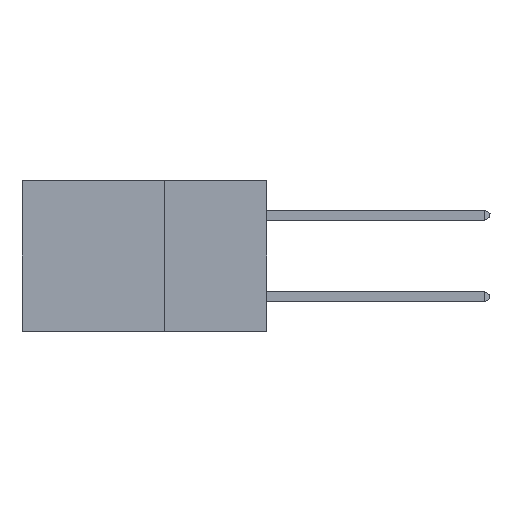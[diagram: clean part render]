
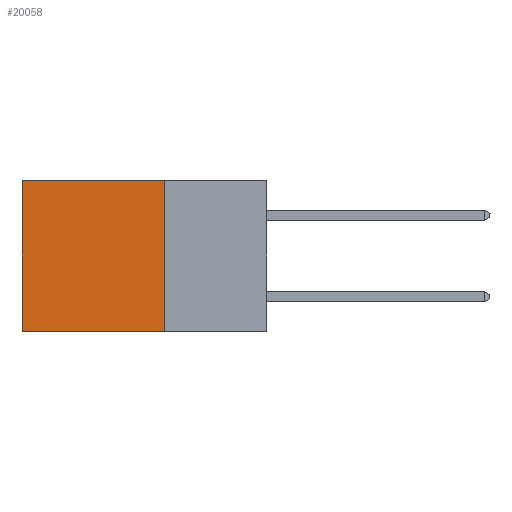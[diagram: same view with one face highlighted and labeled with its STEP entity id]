
A CAD part, left-side view. The second image highlights one B-rep face of the part: STEP entity #20058.
In plain terms, the highlighted planar face has unit normal (-1, 0, 0).
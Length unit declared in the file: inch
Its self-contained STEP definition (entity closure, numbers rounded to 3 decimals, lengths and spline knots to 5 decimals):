
#568 = DIRECTION ( 'NONE',  ( 0., 1., 0. ) ) ;
#647 = DIRECTION ( 'NONE',  ( 0., 0., -1. ) ) ;
#1772 = VECTOR ( 'NONE', #647, 39.37008 ) ;
#4211 = CARTESIAN_POINT ( 'NONE',  ( 0.2875, 0.6, -0.37 ) ) ;
#5570 = LINE ( 'NONE', #9951, #12906 ) ;
#5757 = CARTESIAN_POINT ( 'NONE',  ( 0.2875, 0.6, 0. ) ) ;
#6452 = VERTEX_POINT ( 'NONE', #14968 ) ;
#7390 = EDGE_CURVE ( 'NONE', #19542, #6452, #9391, .T. ) ;
#8199 = EDGE_CURVE ( 'NONE', #23966, #14030, #10862, .T. ) ;
#8934 = ORIENTED_EDGE ( 'NONE', *, *, #8199, .T. ) ;
#9391 = LINE ( 'NONE', #22132, #22801 ) ;
#9604 = LINE ( 'NONE', #13961, #15736 ) ;
#9951 = CARTESIAN_POINT ( 'NONE',  ( 0.2875, 0.25, 0. ) ) ;
#10031 = DIRECTION ( 'NONE',  ( 0., 1., 0. ) ) ;
#10465 = DIRECTION ( 'NONE',  ( 0., 0., -1. ) ) ;
#10862 = LINE ( 'NONE', #5757, #1772 ) ;
#12906 = VECTOR ( 'NONE', #10031, 39.37008 ) ;
#13684 = PLANE ( 'NONE',  #19231 ) ;
#13961 = CARTESIAN_POINT ( 'NONE',  ( 0.2875, 0.25, -0.37 ) ) ;
#14030 = VERTEX_POINT ( 'NONE', #4211 ) ;
#14968 = CARTESIAN_POINT ( 'NONE',  ( 0.2875, 0.25, -0.37 ) ) ;
#15736 = VECTOR ( 'NONE', #568, 39.37008 ) ;
#16479 = EDGE_CURVE ( 'NONE', #6452, #14030, #9604, .T. ) ;
#18958 = ORIENTED_EDGE ( 'NONE', *, *, #7390, .F. ) ;
#19231 = AXIS2_PLACEMENT_3D ( 'NONE', #19682, #19513, #21625 ) ;
#19513 = DIRECTION ( 'NONE',  ( 1., 0., 0. ) ) ;
#19542 = VERTEX_POINT ( 'NONE', #24028 ) ;
#19682 = CARTESIAN_POINT ( 'NONE',  ( 0.2875, 0.25, 0. ) ) ;
#20058 = ADVANCED_FACE ( 'NONE', ( #20972 ), #13684, .F. ) ;
#20972 = FACE_OUTER_BOUND ( 'NONE', #23046, .T. ) ;
#21053 = CARTESIAN_POINT ( 'NONE',  ( 0.2875, 0.6, 0. ) ) ;
#21625 = DIRECTION ( 'NONE',  ( 0., 0., -1. ) ) ;
#22132 = CARTESIAN_POINT ( 'NONE',  ( 0.2875, 0.25, 0. ) ) ;
#22464 = ORIENTED_EDGE ( 'NONE', *, *, #16479, .F. ) ;
#22801 = VECTOR ( 'NONE', #10465, 39.37008 ) ;
#23046 = EDGE_LOOP ( 'NONE', ( #8934, #22464, #18958, #23152 ) ) ;
#23152 = ORIENTED_EDGE ( 'NONE', *, *, #24842, .T. ) ;
#23966 = VERTEX_POINT ( 'NONE', #21053 ) ;
#24028 = CARTESIAN_POINT ( 'NONE',  ( 0.2875, 0.25, 0. ) ) ;
#24842 = EDGE_CURVE ( 'NONE', #19542, #23966, #5570, .T. ) ;
